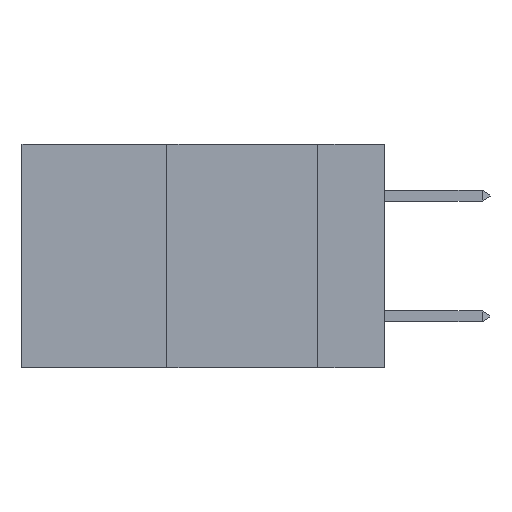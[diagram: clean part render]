
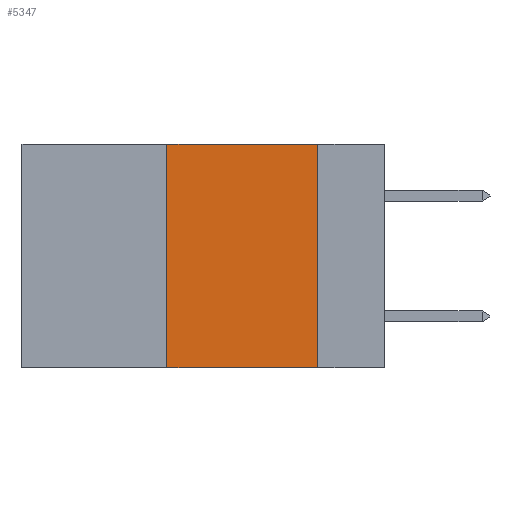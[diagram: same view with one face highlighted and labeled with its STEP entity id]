
A CAD part, left-side view. The second image highlights one B-rep face of the part: STEP entity #5347.
In plain terms, the highlighted planar face has unit normal (-1, 0, 0).
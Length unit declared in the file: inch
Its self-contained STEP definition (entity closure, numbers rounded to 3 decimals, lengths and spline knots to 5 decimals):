
#1285 = LINE ( 'NONE', #14347, #32549 ) ;
#1625 = DIRECTION ( 'NONE',  ( 0., 0., 1. ) ) ;
#2201 = DIRECTION ( 'NONE',  ( 0., -1., 0. ) ) ;
#3272 = VECTOR ( 'NONE', #2201, 39.37008 ) ;
#3396 = ORIENTED_EDGE ( 'NONE', *, *, #29235, .F. ) ;
#5088 = DIRECTION ( 'NONE',  ( 0., 0., -1. ) ) ;
#5199 = DIRECTION ( 'NONE',  ( 0., -1., 0. ) ) ;
#5347 = ADVANCED_FACE ( 'NONE', ( #9319 ), #19513, .F. ) ;
#7483 = ORIENTED_EDGE ( 'NONE', *, *, #31844, .T. ) ;
#7613 = CARTESIAN_POINT ( 'NONE',  ( 0., 0.11, 0. ) ) ;
#9319 = FACE_OUTER_BOUND ( 'NONE', #20904, .T. ) ;
#9982 = VERTEX_POINT ( 'NONE', #17622 ) ;
#10516 = VERTEX_POINT ( 'NONE', #26346 ) ;
#11594 = VERTEX_POINT ( 'NONE', #16767 ) ;
#12305 = LINE ( 'NONE', #7613, #19816 ) ;
#14026 = ORIENTED_EDGE ( 'NONE', *, *, #16495, .F. ) ;
#14347 = CARTESIAN_POINT ( 'NONE',  ( 0., 0.36, 0. ) ) ;
#14665 = DIRECTION ( 'NONE',  ( 1., 0., 0. ) ) ;
#14738 = LINE ( 'NONE', #25900, #24051 ) ;
#16495 = EDGE_CURVE ( 'NONE', #9982, #10516, #1285, .T. ) ;
#16767 = CARTESIAN_POINT ( 'NONE',  ( 0., 0.11, 0. ) ) ;
#17622 = CARTESIAN_POINT ( 'NONE',  ( 0., 0.36, -0.37 ) ) ;
#19357 = DIRECTION ( 'NONE',  ( 0., 0., -1. ) ) ;
#19513 = PLANE ( 'NONE',  #23603 ) ;
#19539 = CARTESIAN_POINT ( 'NONE',  ( 0., 0.11, -0.37 ) ) ;
#19777 = LINE ( 'NONE', #32778, #3272 ) ;
#19816 = VECTOR ( 'NONE', #5088, 39.37008 ) ;
#20034 = ORIENTED_EDGE ( 'NONE', *, *, #31372, .F. ) ;
#20904 = EDGE_LOOP ( 'NONE', ( #20034, #3396, #14026, #7483 ) ) ;
#23603 = AXIS2_PLACEMENT_3D ( 'NONE', #32355, #14665, #19357 ) ;
#24051 = VECTOR ( 'NONE', #5199, 39.37008 ) ;
#25237 = VERTEX_POINT ( 'NONE', #19539 ) ;
#25900 = CARTESIAN_POINT ( 'NONE',  ( 0., 0.6, 0. ) ) ;
#26346 = CARTESIAN_POINT ( 'NONE',  ( 0., 0.36, 0. ) ) ;
#29235 = EDGE_CURVE ( 'NONE', #10516, #11594, #14738, .T. ) ;
#31372 = EDGE_CURVE ( 'NONE', #11594, #25237, #12305, .T. ) ;
#31844 = EDGE_CURVE ( 'NONE', #9982, #25237, #19777, .T. ) ;
#32355 = CARTESIAN_POINT ( 'NONE',  ( 0., 0.6, 0. ) ) ;
#32549 = VECTOR ( 'NONE', #1625, 39.37008 ) ;
#32778 = CARTESIAN_POINT ( 'NONE',  ( 0., 0.6, -0.37 ) ) ;
